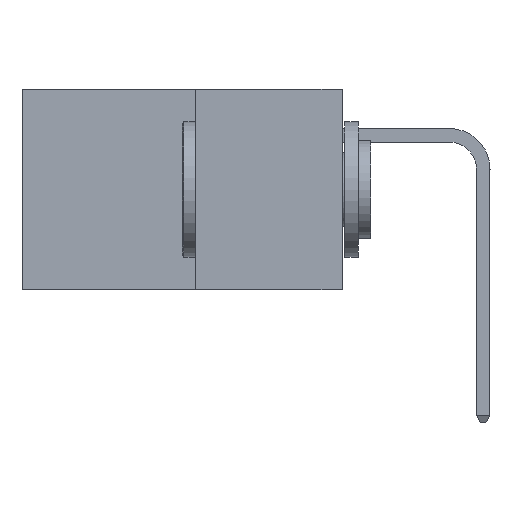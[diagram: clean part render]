
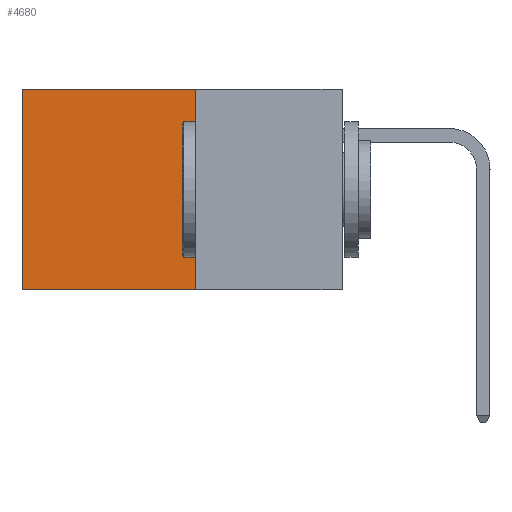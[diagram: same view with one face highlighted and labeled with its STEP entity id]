
A CAD part, left-side view. The second image highlights one B-rep face of the part: STEP entity #4680.
In plain terms, the highlighted planar face has unit normal (-1, 0, 0).
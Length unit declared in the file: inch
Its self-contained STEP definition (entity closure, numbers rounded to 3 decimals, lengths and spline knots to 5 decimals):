
#745 = ORIENTED_EDGE ( 'NONE', *, *, #10740, .T. ) ;
#1038 = CARTESIAN_POINT ( 'NONE',  ( 0.277, 0.59, 0. ) ) ;
#1285 = DIRECTION ( 'NONE',  ( 0., 0., -1. ) ) ;
#1589 = CARTESIAN_POINT ( 'NONE',  ( 0.277, 0.27, -0.37 ) ) ;
#2475 = VERTEX_POINT ( 'NONE', #25621 ) ;
#2740 = EDGE_CURVE ( 'NONE', #2475, #9408, #16442, .T. ) ;
#3844 = ORIENTED_EDGE ( 'NONE', *, *, #20247, .F. ) ;
#4263 = CARTESIAN_POINT ( 'NONE',  ( 0.277, 0.27, -0.37 ) ) ;
#4460 = CARTESIAN_POINT ( 'NONE',  ( 0.277, 0.27, -0.37 ) ) ;
#4548 = EDGE_CURVE ( 'NONE', #2475, #18409, #19303, .T. ) ;
#4680 = ADVANCED_FACE ( 'NONE', ( #20934 ), #24345, .F. ) ;
#6239 = ORIENTED_EDGE ( 'NONE', *, *, #4548, .F. ) ;
#6937 = AXIS2_PLACEMENT_3D ( 'NONE', #24151, #24061, #24027 ) ;
#7801 = LINE ( 'NONE', #4460, #8461 ) ;
#8461 = VECTOR ( 'NONE', #21223, 39.37008 ) ;
#9408 = VERTEX_POINT ( 'NONE', #1038 ) ;
#10140 = VECTOR ( 'NONE', #17878, 39.37008 ) ;
#10740 = EDGE_CURVE ( 'NONE', #9408, #17719, #26903, .T. ) ;
#15162 = VECTOR ( 'NONE', #19698, 39.37008 ) ;
#15769 = CARTESIAN_POINT ( 'NONE',  ( 0.277, 0.59, -0.37 ) ) ;
#16442 = LINE ( 'NONE', #20073, #15162 ) ;
#17719 = VERTEX_POINT ( 'NONE', #25092 ) ;
#17878 = DIRECTION ( 'NONE',  ( 0., 0., -1. ) ) ;
#18409 = VERTEX_POINT ( 'NONE', #4263 ) ;
#19303 = LINE ( 'NONE', #1589, #19964 ) ;
#19698 = DIRECTION ( 'NONE',  ( 0., 1., 0. ) ) ;
#19964 = VECTOR ( 'NONE', #1285, 39.37008 ) ;
#20073 = CARTESIAN_POINT ( 'NONE',  ( 0.277, 0.27, 0. ) ) ;
#20247 = EDGE_CURVE ( 'NONE', #18409, #17719, #7801, .T. ) ;
#20934 = FACE_OUTER_BOUND ( 'NONE', #24624, .T. ) ;
#21223 = DIRECTION ( 'NONE',  ( 0., 1., 0. ) ) ;
#23412 = ORIENTED_EDGE ( 'NONE', *, *, #2740, .T. ) ;
#24027 = DIRECTION ( 'NONE',  ( 0., 0., -1. ) ) ;
#24061 = DIRECTION ( 'NONE',  ( 1., 0., 0. ) ) ;
#24151 = CARTESIAN_POINT ( 'NONE',  ( 0.277, 0.27, -0.37 ) ) ;
#24345 = PLANE ( 'NONE',  #6937 ) ;
#24624 = EDGE_LOOP ( 'NONE', ( #745, #3844, #6239, #23412 ) ) ;
#25092 = CARTESIAN_POINT ( 'NONE',  ( 0.277, 0.59, -0.37 ) ) ;
#25621 = CARTESIAN_POINT ( 'NONE',  ( 0.277, 0.27, 0. ) ) ;
#26903 = LINE ( 'NONE', #15769, #10140 ) ;
